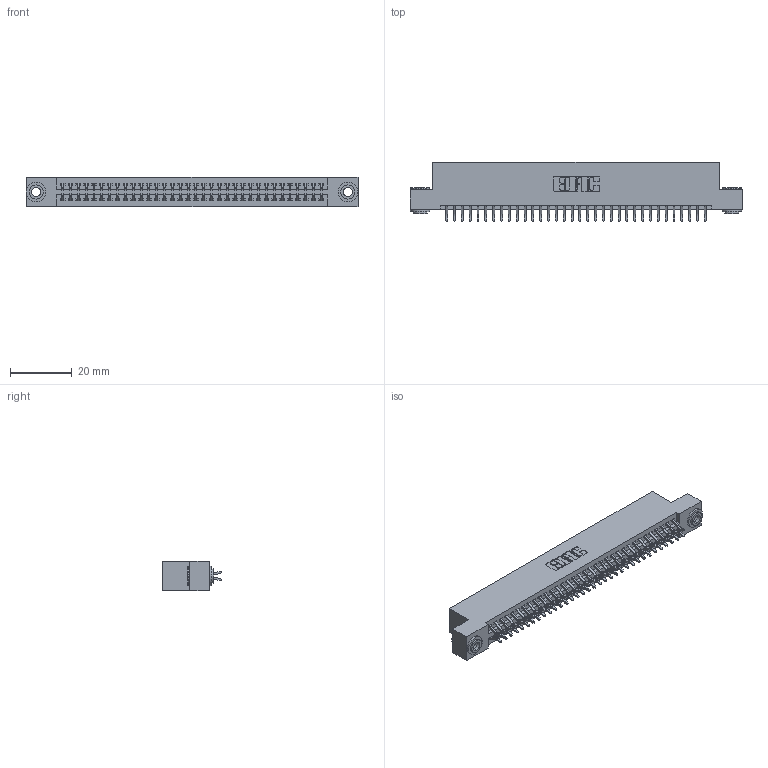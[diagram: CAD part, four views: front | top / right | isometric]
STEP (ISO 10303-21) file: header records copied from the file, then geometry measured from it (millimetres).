
FILE_DESCRIPTION (( 'STEP AP203' ), '1' );
FILE_NAME ('395-068-556-203.STEP', '2018-11-25T18:53:07', ( '' ), ( '' ), 'SwSTEP 2.0', 'SolidWorks 2016', '' );
FILE_SCHEMA (( 'CONFIG_CONTROL_DESIGN' ));
Length unit declared in the file: inch
Products named in the file (4): 345-250-002_345-250-002-102; 395-068-556-203; 345 Part_Flush Mounting Lugs - 0.156 Dia-TH; 345-292-001_556 Tail
Assembly tree (71 placements, depth 2):
  395-068-556-203
    345 Part_Flush Mounting Lugs - 0.156 Dia-TH
    345-292-001_556 Tail  x68
    345-250-002_345-250-002-102  x2
Bounding box: 107.57 x 19.24 x 9.4 mm (x, y, z)
Volume: 10391.8 mm3; surface area: 15351.3 mm2
Topology: 71 solids, 71 shells, 3972 faces, 11773 edges, 7754 vertices
Faces by surface type: plane 2606, cylinder 1358, cone 8
Entity records: 28624 total; most frequent: CARTESIAN_POINT 4795, ORIENTED_EDGE 4710, DIRECTION 4257, EDGE_CURVE 2355, VECTOR 2055, LINE 2055, VERTEX_POINT 1566, AXIS2_PLACEMENT_3D 1101
